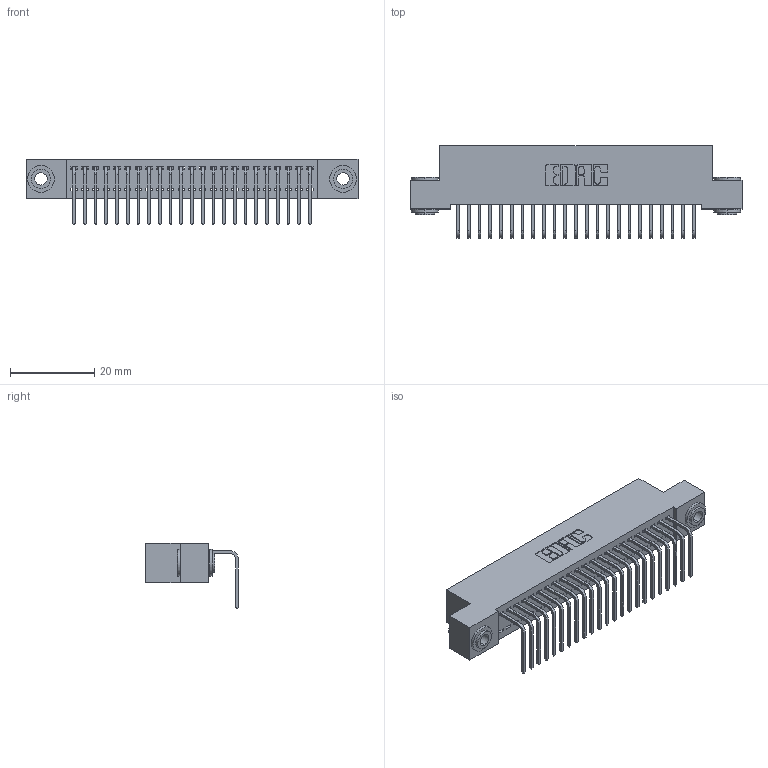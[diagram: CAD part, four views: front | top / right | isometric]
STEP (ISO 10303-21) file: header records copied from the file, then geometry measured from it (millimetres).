
FILE_DESCRIPTION (( 'STEP AP203' ), '1' );
FILE_NAME ('392-023-558-103.STEP', '2019-10-07T07:00:22', ( '' ), ( '' ), 'SwSTEP 2.0', 'SolidWorks 2016', '' );
FILE_SCHEMA (( 'CONFIG_CONTROL_DESIGN' ));
Length unit declared in the file: inch
Products named in the file (4): 392-023-558-103; 342 Part_.156 TH; 345-292-001_558 Tail - 2; 342-250-002_345-250-002-102
Assembly tree (26 placements, depth 2):
  392-023-558-103
    342 Part_.156 TH
    345-292-001_558 Tail - 2  x23
    342-250-002_345-250-002-102  x2
Bounding box: 78.74 x 21.91 x 15.62 mm (x, y, z)
Volume: 6933.4 mm3; surface area: 10488 mm2
Topology: 26 solids, 26 shells, 1528 faces, 4561 edges, 3006 vertices
Faces by surface type: plane 1088, cylinder 432, cone 8
Entity records: 17120 total; most frequent: CARTESIAN_POINT 2934, ORIENTED_EDGE 2886, DIRECTION 2547, EDGE_CURVE 1443, VECTOR 1291, LINE 1291, VERTEX_POINT 958, AXIS2_PLACEMENT_3D 628
